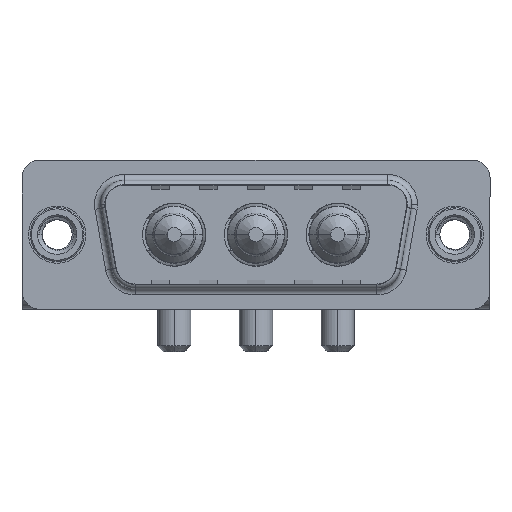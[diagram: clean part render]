
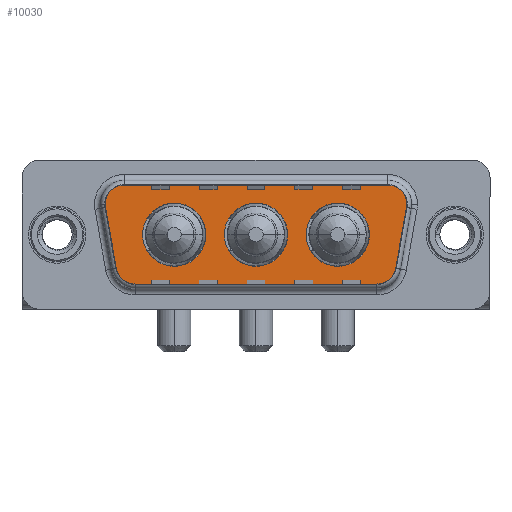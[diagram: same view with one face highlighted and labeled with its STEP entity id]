
A CAD part, top view. The second image highlights one B-rep face of the part: STEP entity #10030.
In plain terms, the highlighted planar face has unit normal (0, 0, 1).
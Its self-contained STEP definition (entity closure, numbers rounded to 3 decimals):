
#66 = CARTESIAN_POINT ( 'NONE',  ( 27.889, 4.9, 0. ) ) ;
#97 = AXIS2_PLACEMENT_3D ( 'NONE', #11988, #14386, #2633 ) ;
#112 = EDGE_CURVE ( 'NONE', #4568, #14999, #14312, .T. ) ;
#230 = CARTESIAN_POINT ( 'NONE',  ( 14., 0., 0. ) ) ;
#347 = ORIENTED_EDGE ( 'NONE', *, *, #6528, .T. ) ;
#482 = VERTEX_POINT ( 'NONE', #4771 ) ;
#496 = ORIENTED_EDGE ( 'NONE', *, *, #13646, .T. ) ;
#557 = FACE_BOUND ( 'NONE', #13300, .T. ) ;
#575 = DIRECTION ( 'NONE',  ( 0., 0., 1. ) ) ;
#820 = CARTESIAN_POINT ( 'NONE',  ( 23.5, 0., 0. ) ) ;
#868 = EDGE_LOOP ( 'NONE', ( #6705, #4934 ) ) ;
#957 = CARTESIAN_POINT ( 'NONE',  ( 26.866, -4.9, 0. ) ) ;
#981 = ORIENTED_EDGE ( 'NONE', *, *, #9002, .F. ) ;
#1226 = EDGE_CURVE ( 'NONE', #4612, #2183, #15365, .T. ) ;
#1248 = VERTEX_POINT ( 'NONE', #9448 ) ;
#1259 = VERTEX_POINT ( 'NONE', #3526 ) ;
#1606 = CARTESIAN_POINT ( 'NONE',  ( 27.889, 2.9, 0. ) ) ;
#1817 = DIRECTION ( 'NONE',  ( 1., 0., 0. ) ) ;
#2183 = VERTEX_POINT ( 'NONE', #10049 ) ;
#2217 = EDGE_CURVE ( 'NONE', #5221, #4568, #7931, .T. ) ;
#2633 = DIRECTION ( 'NONE',  ( -1., 0., 0. ) ) ;
#2753 = CIRCLE ( 'NONE', #4498, 2.65 ) ;
#2767 = ORIENTED_EDGE ( 'NONE', *, *, #10359, .T. ) ;
#2772 = DIRECTION ( 'NONE',  ( 0., 0., 1. ) ) ;
#2850 = DIRECTION ( 'NONE',  ( 0.174, -0.985, 0. ) ) ;
#3048 = PLANE ( 'NONE',  #14080 ) ;
#3054 = DIRECTION ( 'NONE',  ( 1., 0., 0. ) ) ;
#3128 = CARTESIAN_POINT ( 'NONE',  ( 9.8, 0., 0. ) ) ;
#3246 = DIRECTION ( 'NONE',  ( 0.174, 0.985, 0. ) ) ;
#3360 = VERTEX_POINT ( 'NONE', #957 ) ;
#3526 = CARTESIAN_POINT ( 'NONE',  ( 29.889, 2.9, 0. ) ) ;
#3784 = CARTESIAN_POINT ( 'NONE',  ( 5.411, 2.9, 0. ) ) ;
#3788 = EDGE_CURVE ( 'NONE', #14894, #14612, #6087, .T. ) ;
#3807 = DIRECTION ( 'NONE',  ( 0., 0., 1. ) ) ;
#4078 = DIRECTION ( 'NONE',  ( 0., 0., 1. ) ) ;
#4087 = DIRECTION ( 'NONE',  ( 1., 0., 0. ) ) ;
#4120 = EDGE_CURVE ( 'NONE', #14612, #3360, #4502, .T. ) ;
#4372 = CARTESIAN_POINT ( 'NONE',  ( 23.5, 0., 0. ) ) ;
#4498 = AXIS2_PLACEMENT_3D ( 'NONE', #14662, #575, #4087 ) ;
#4502 = LINE ( 'NONE', #12686, #13524 ) ;
#4568 = VERTEX_POINT ( 'NONE', #7669 ) ;
#4612 = VERTEX_POINT ( 'NONE', #5258 ) ;
#4771 = CARTESIAN_POINT ( 'NONE',  ( 7.15, 0., 0. ) ) ;
#4933 = CARTESIAN_POINT ( 'NONE',  ( 27.889, 2.9, 0. ) ) ;
#4934 = ORIENTED_EDGE ( 'NONE', *, *, #9403, .F. ) ;
#5127 = LINE ( 'NONE', #8863, #9920 ) ;
#5175 = CIRCLE ( 'NONE', #11120, 2.65 ) ;
#5182 = ORIENTED_EDGE ( 'NONE', *, *, #10607, .F. ) ;
#5221 = VERTEX_POINT ( 'NONE', #66 ) ;
#5236 = DIRECTION ( 'NONE',  ( -1., 0., 0. ) ) ;
#5258 = CARTESIAN_POINT ( 'NONE',  ( 28.836, -3.247, 0. ) ) ;
#5268 = EDGE_CURVE ( 'NONE', #3360, #4612, #9865, .T. ) ;
#5898 = AXIS2_PLACEMENT_3D ( 'NONE', #3128, #9052, #3054 ) ;
#5910 = CIRCLE ( 'NONE', #11107, 2. ) ;
#5918 = DIRECTION ( 'NONE',  ( 0., 0., 1. ) ) ;
#6087 = CIRCLE ( 'NONE', #97, 2. ) ;
#6317 = CARTESIAN_POINT ( 'NONE',  ( 5.411, 4.9, 0. ) ) ;
#6355 = ORIENTED_EDGE ( 'NONE', *, *, #3788, .T. ) ;
#6528 = EDGE_CURVE ( 'NONE', #1259, #5221, #7058, .T. ) ;
#6645 = CARTESIAN_POINT ( 'NONE',  ( 4.464, -3.247, 0. ) ) ;
#6683 = CARTESIAN_POINT ( 'NONE',  ( 29.859, 2.553, 0. ) ) ;
#6705 = ORIENTED_EDGE ( 'NONE', *, *, #11749, .F. ) ;
#6778 = FACE_OUTER_BOUND ( 'NONE', #10311, .T. ) ;
#6853 = AXIS2_PLACEMENT_3D ( 'NONE', #3784, #4078, #1817 ) ;
#7058 = CIRCLE ( 'NONE', #7823, 2. ) ;
#7222 = ORIENTED_EDGE ( 'NONE', *, *, #5268, .T. ) ;
#7367 = EDGE_CURVE ( 'NONE', #12055, #12476, #2753, .T. ) ;
#7390 = ORIENTED_EDGE ( 'NONE', *, *, #4120, .T. ) ;
#7669 = CARTESIAN_POINT ( 'NONE',  ( 5.411, 4.9, 0. ) ) ;
#7721 = DIRECTION ( 'NONE',  ( 0., 0., 1. ) ) ;
#7823 = AXIS2_PLACEMENT_3D ( 'NONE', #4933, #12074, #9673 ) ;
#7931 = LINE ( 'NONE', #6317, #9740 ) ;
#8107 = AXIS2_PLACEMENT_3D ( 'NONE', #10996, #14263, #13188 ) ;
#8465 = CARTESIAN_POINT ( 'NONE',  ( 12.45, 0., 0. ) ) ;
#8612 = CARTESIAN_POINT ( 'NONE',  ( 16.65, 0., 0. ) ) ;
#8857 = DIRECTION ( 'NONE',  ( -1., 0., 0. ) ) ;
#8863 = CARTESIAN_POINT ( 'NONE',  ( 3.441, 2.553, 0. ) ) ;
#9002 = EDGE_CURVE ( 'NONE', #12476, #12055, #5175, .T. ) ;
#9047 = DIRECTION ( 'NONE',  ( 1., 0., 0. ) ) ;
#9052 = DIRECTION ( 'NONE',  ( 0., 0., 1. ) ) ;
#9116 = ORIENTED_EDGE ( 'NONE', *, *, #2217, .T. ) ;
#9126 = FACE_BOUND ( 'NONE', #868, .T. ) ;
#9403 = EDGE_CURVE ( 'NONE', #482, #13926, #15104, .T. ) ;
#9448 = CARTESIAN_POINT ( 'NONE',  ( 26.15, 0., 0. ) ) ;
#9673 = DIRECTION ( 'NONE',  ( -1., 0., 0. ) ) ;
#9740 = VECTOR ( 'NONE', #5236, 1000. ) ;
#9865 = CIRCLE ( 'NONE', #10351, 2. ) ;
#9920 = VECTOR ( 'NONE', #2850, 1000. ) ;
#10020 = EDGE_CURVE ( 'NONE', #1248, #14731, #14324, .T. ) ;
#10030 = ADVANCED_FACE ( 'NONE', ( #557, #13776, #9126, #6778 ), #3048, .T. ) ;
#10049 = CARTESIAN_POINT ( 'NONE',  ( 29.859, 2.553, 0. ) ) ;
#10311 = EDGE_LOOP ( 'NONE', ( #7222, #11053, #2767, #347, #9116, #14869, #496, #6355, #7390 ) ) ;
#10312 = DIRECTION ( 'NONE',  ( 0., 0., 1. ) ) ;
#10351 = AXIS2_PLACEMENT_3D ( 'NONE', #10896, #3807, #12062 ) ;
#10359 = EDGE_CURVE ( 'NONE', #2183, #1259, #5910, .T. ) ;
#10604 = CIRCLE ( 'NONE', #5898, 2.65 ) ;
#10607 = EDGE_CURVE ( 'NONE', #14731, #1248, #11608, .T. ) ;
#10625 = CARTESIAN_POINT ( 'NONE',  ( 19.3, 0., 0. ) ) ;
#10896 = CARTESIAN_POINT ( 'NONE',  ( 26.866, -2.9, 0. ) ) ;
#10922 = CARTESIAN_POINT ( 'NONE',  ( 6.434, -4.9, 0. ) ) ;
#10996 = CARTESIAN_POINT ( 'NONE',  ( 9.8, 0., 0. ) ) ;
#11053 = ORIENTED_EDGE ( 'NONE', *, *, #1226, .T. ) ;
#11107 = AXIS2_PLACEMENT_3D ( 'NONE', #1606, #2772, #8857 ) ;
#11120 = AXIS2_PLACEMENT_3D ( 'NONE', #8612, #5918, #15404 ) ;
#11515 = EDGE_LOOP ( 'NONE', ( #14930, #5182 ) ) ;
#11608 = CIRCLE ( 'NONE', #12362, 2.65 ) ;
#11733 = DIRECTION ( 'NONE',  ( 1., 0., 0. ) ) ;
#11749 = EDGE_CURVE ( 'NONE', #13926, #482, #10604, .T. ) ;
#11988 = CARTESIAN_POINT ( 'NONE',  ( 6.434, -2.9, 0. ) ) ;
#12055 = VERTEX_POINT ( 'NONE', #230 ) ;
#12062 = DIRECTION ( 'NONE',  ( 1., 0., 0. ) ) ;
#12074 = DIRECTION ( 'NONE',  ( 0., 0., 1. ) ) ;
#12362 = AXIS2_PLACEMENT_3D ( 'NONE', #820, #10312, #15061 ) ;
#12475 = CARTESIAN_POINT ( 'NONE',  ( 26.866, -2.9, 0. ) ) ;
#12476 = VERTEX_POINT ( 'NONE', #10625 ) ;
#12635 = DIRECTION ( 'NONE',  ( 0., 0., 1. ) ) ;
#12686 = CARTESIAN_POINT ( 'NONE',  ( 6.434, -4.9, 0. ) ) ;
#12778 = CARTESIAN_POINT ( 'NONE',  ( 3.441, 2.553, 0. ) ) ;
#13114 = VECTOR ( 'NONE', #3246, 1000. ) ;
#13188 = DIRECTION ( 'NONE',  ( 1., 0., 0. ) ) ;
#13300 = EDGE_LOOP ( 'NONE', ( #981, #13974 ) ) ;
#13524 = VECTOR ( 'NONE', #11733, 1000. ) ;
#13634 = DIRECTION ( 'NONE',  ( 1., 0., 0. ) ) ;
#13646 = EDGE_CURVE ( 'NONE', #14999, #14894, #5127, .T. ) ;
#13718 = CARTESIAN_POINT ( 'NONE',  ( 20.85, 0., 0. ) ) ;
#13776 = FACE_BOUND ( 'NONE', #11515, .T. ) ;
#13826 = AXIS2_PLACEMENT_3D ( 'NONE', #4372, #7721, #9047 ) ;
#13926 = VERTEX_POINT ( 'NONE', #8465 ) ;
#13974 = ORIENTED_EDGE ( 'NONE', *, *, #7367, .F. ) ;
#14080 = AXIS2_PLACEMENT_3D ( 'NONE', #12475, #12635, #13634 ) ;
#14263 = DIRECTION ( 'NONE',  ( 0., 0., 1. ) ) ;
#14312 = CIRCLE ( 'NONE', #6853, 2. ) ;
#14324 = CIRCLE ( 'NONE', #13826, 2.65 ) ;
#14386 = DIRECTION ( 'NONE',  ( 0., 0., 1. ) ) ;
#14612 = VERTEX_POINT ( 'NONE', #10922 ) ;
#14662 = CARTESIAN_POINT ( 'NONE',  ( 16.65, 0., 0. ) ) ;
#14731 = VERTEX_POINT ( 'NONE', #13718 ) ;
#14869 = ORIENTED_EDGE ( 'NONE', *, *, #112, .T. ) ;
#14894 = VERTEX_POINT ( 'NONE', #6645 ) ;
#14930 = ORIENTED_EDGE ( 'NONE', *, *, #10020, .F. ) ;
#14999 = VERTEX_POINT ( 'NONE', #12778 ) ;
#15061 = DIRECTION ( 'NONE',  ( 1., 0., 0. ) ) ;
#15104 = CIRCLE ( 'NONE', #8107, 2.65 ) ;
#15365 = LINE ( 'NONE', #6683, #13114 ) ;
#15404 = DIRECTION ( 'NONE',  ( 1., 0., 0. ) ) ;
